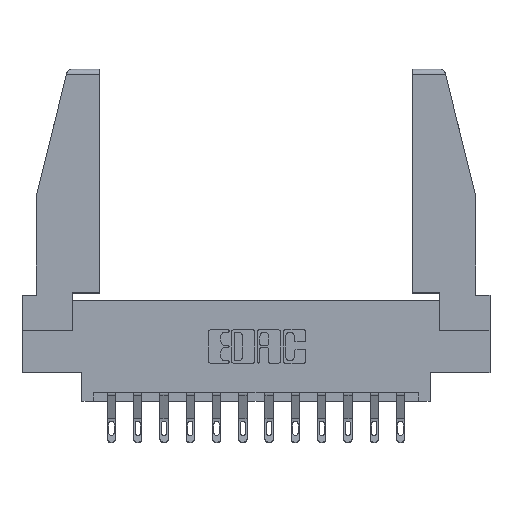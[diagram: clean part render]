
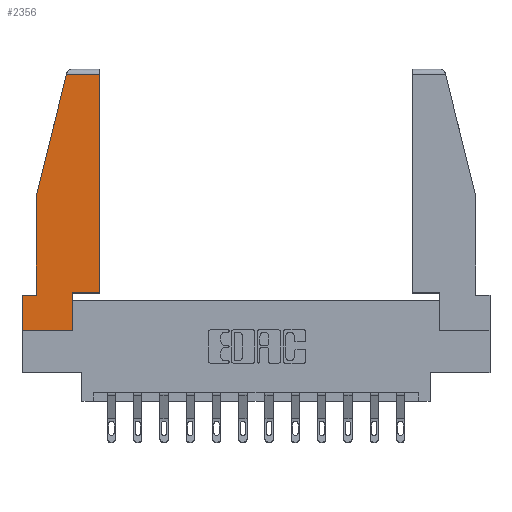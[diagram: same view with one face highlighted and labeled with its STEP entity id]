
A CAD part, top view. The second image highlights one B-rep face of the part: STEP entity #2356.
In plain terms, the highlighted planar face has unit normal (0, 0, 1).
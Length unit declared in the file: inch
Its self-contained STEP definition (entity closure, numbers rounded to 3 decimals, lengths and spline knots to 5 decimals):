
#3 = EDGE_LOOP ( 'NONE', ( #10482, #5700, #3877, #15354, #9767, #13825, #12193, #12613, #4576 ) ) ;
#454 = CARTESIAN_POINT ( 'NONE',  ( 0., 0.21, 0. ) ) ;
#768 = DIRECTION ( 'NONE',  ( 0., -1., 0. ) ) ;
#878 = EDGE_CURVE ( 'NONE', #14418, #12314, #13923, .T. ) ;
#1473 = CARTESIAN_POINT ( 'NONE',  ( 0.086, 0.8, 0. ) ) ;
#1529 = LINE ( 'NONE', #11196, #15495 ) ;
#1798 = EDGE_CURVE ( 'NONE', #6936, #5879, #16043, .T. ) ;
#2188 = EDGE_CURVE ( 'NONE', #2968, #4499, #11132, .T. ) ;
#2258 = CARTESIAN_POINT ( 'NONE',  ( 0.086, 0.8, 0. ) ) ;
#2356 = ADVANCED_FACE ( 'NONE', ( #8836 ), #11055, .T. ) ;
#2464 = VECTOR ( 'NONE', #15035, 39.37008 ) ;
#2968 = VERTEX_POINT ( 'NONE', #6735 ) ;
#3608 = DIRECTION ( 'NONE',  ( 0., 0., 1. ) ) ;
#3738 = DIRECTION ( 'NONE',  ( 0., 1., 0. ) ) ;
#3877 = ORIENTED_EDGE ( 'NONE', *, *, #14933, .T. ) ;
#4499 = VERTEX_POINT ( 'NONE', #7654 ) ;
#4576 = ORIENTED_EDGE ( 'NONE', *, *, #6029, .T. ) ;
#4744 = VECTOR ( 'NONE', #768, 39.37008 ) ;
#5126 = VECTOR ( 'NONE', #8283, 39.37008 ) ;
#5683 = CARTESIAN_POINT ( 'NONE',  ( 0.297, 0., 0. ) ) ;
#5700 = ORIENTED_EDGE ( 'NONE', *, *, #2188, .T. ) ;
#5879 = VERTEX_POINT ( 'NONE', #5683 ) ;
#6029 = EDGE_CURVE ( 'NONE', #13261, #15563, #7944, .T. ) ;
#6175 = DIRECTION ( 'NONE',  ( 1., 0., 0. ) ) ;
#6311 = CARTESIAN_POINT ( 'NONE',  ( 0.461, 0.223, 0. ) ) ;
#6343 = CARTESIAN_POINT ( 'NONE',  ( 0., 0., 0. ) ) ;
#6354 = LINE ( 'NONE', #11724, #12128 ) ;
#6428 = LINE ( 'NONE', #10278, #15936 ) ;
#6735 = CARTESIAN_POINT ( 'NONE',  ( 0.461, 1.52, 0. ) ) ;
#6936 = VERTEX_POINT ( 'NONE', #14881 ) ;
#7518 = CARTESIAN_POINT ( 'NONE',  ( 0.297, 0.223, 0. ) ) ;
#7654 = CARTESIAN_POINT ( 'NONE',  ( 0.2636, 1.52, 0. ) ) ;
#7901 = LINE ( 'NONE', #454, #4744 ) ;
#7944 = LINE ( 'NONE', #10290, #13952 ) ;
#8019 = EDGE_CURVE ( 'NONE', #8057, #6936, #7901, .T. ) ;
#8025 = EDGE_CURVE ( 'NONE', #12314, #8057, #13698, .T. ) ;
#8057 = VERTEX_POINT ( 'NONE', #10524 ) ;
#8283 = DIRECTION ( 'NONE',  ( -1., 0., 0. ) ) ;
#8836 = FACE_OUTER_BOUND ( 'NONE', #3, .T. ) ;
#9265 = CARTESIAN_POINT ( 'NONE',  ( 0., 0.21, 0. ) ) ;
#9468 = CARTESIAN_POINT ( 'NONE',  ( 0., 1.52, 0. ) ) ;
#9767 = ORIENTED_EDGE ( 'NONE', *, *, #8025, .T. ) ;
#9858 = EDGE_CURVE ( 'NONE', #15563, #2968, #1529, .T. ) ;
#9920 = AXIS2_PLACEMENT_3D ( 'NONE', #14645, #3608, #10836 ) ;
#10278 = CARTESIAN_POINT ( 'NONE',  ( 0.297, 0., 0. ) ) ;
#10290 = CARTESIAN_POINT ( 'NONE',  ( 0.297, 0.223, 0. ) ) ;
#10380 = VECTOR ( 'NONE', #14284, 39.37008 ) ;
#10482 = ORIENTED_EDGE ( 'NONE', *, *, #9858, .T. ) ;
#10524 = CARTESIAN_POINT ( 'NONE',  ( 0., 0.21, 0. ) ) ;
#10836 = DIRECTION ( 'NONE',  ( 1., 0., 0. ) ) ;
#11055 = PLANE ( 'NONE',  #9920 ) ;
#11132 = LINE ( 'NONE', #9468, #5126 ) ;
#11196 = CARTESIAN_POINT ( 'NONE',  ( 0.461, 0.223, 0. ) ) ;
#11724 = CARTESIAN_POINT ( 'NONE',  ( 0.271, 1.55, 0. ) ) ;
#12128 = VECTOR ( 'NONE', #15337, 39.37008 ) ;
#12193 = ORIENTED_EDGE ( 'NONE', *, *, #1798, .T. ) ;
#12314 = VERTEX_POINT ( 'NONE', #13770 ) ;
#12613 = ORIENTED_EDGE ( 'NONE', *, *, #15961, .T. ) ;
#13261 = VERTEX_POINT ( 'NONE', #7518 ) ;
#13698 = LINE ( 'NONE', #9265, #10380 ) ;
#13770 = CARTESIAN_POINT ( 'NONE',  ( 0.086, 0.21, 0. ) ) ;
#13825 = ORIENTED_EDGE ( 'NONE', *, *, #8019, .T. ) ;
#13923 = LINE ( 'NONE', #1473, #2464 ) ;
#13946 = DIRECTION ( 'NONE',  ( 1., 0., 0. ) ) ;
#13952 = VECTOR ( 'NONE', #13946, 39.37008 ) ;
#13982 = DIRECTION ( 'NONE',  ( 0., 1., 0. ) ) ;
#14284 = DIRECTION ( 'NONE',  ( -1., 0., 0. ) ) ;
#14418 = VERTEX_POINT ( 'NONE', #2258 ) ;
#14451 = VECTOR ( 'NONE', #6175, 39.37008 ) ;
#14645 = CARTESIAN_POINT ( 'NONE',  ( 0., 0., 0. ) ) ;
#14881 = CARTESIAN_POINT ( 'NONE',  ( 0., 0., 0. ) ) ;
#14933 = EDGE_CURVE ( 'NONE', #4499, #14418, #6354, .T. ) ;
#15035 = DIRECTION ( 'NONE',  ( 0., -1., 0. ) ) ;
#15337 = DIRECTION ( 'NONE',  ( -0.239, -0.971, 0. ) ) ;
#15354 = ORIENTED_EDGE ( 'NONE', *, *, #878, .T. ) ;
#15495 = VECTOR ( 'NONE', #3738, 39.37008 ) ;
#15563 = VERTEX_POINT ( 'NONE', #6311 ) ;
#15936 = VECTOR ( 'NONE', #13982, 39.37008 ) ;
#15961 = EDGE_CURVE ( 'NONE', #5879, #13261, #6428, .T. ) ;
#16043 = LINE ( 'NONE', #6343, #14451 ) ;
